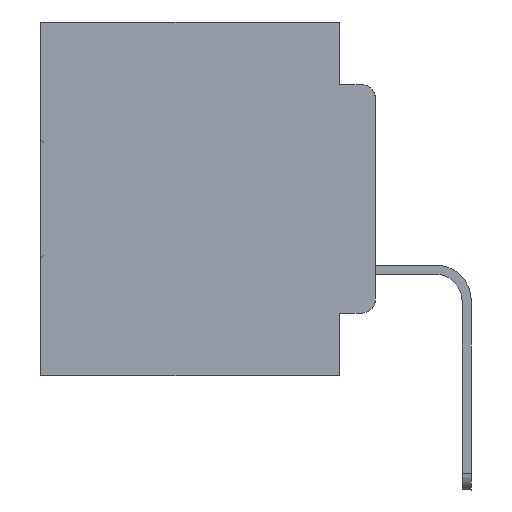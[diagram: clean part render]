
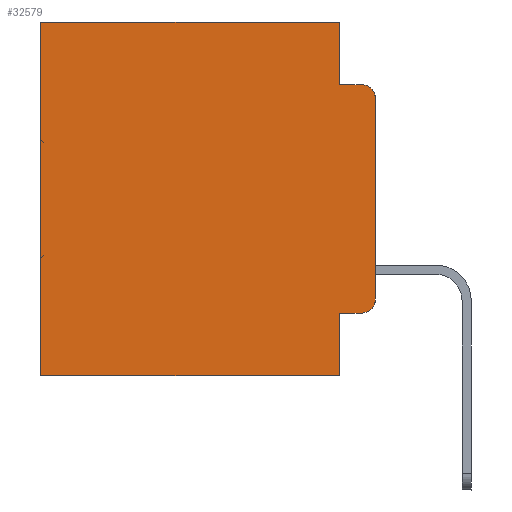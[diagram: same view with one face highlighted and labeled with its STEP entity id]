
A CAD part, left-side view. The second image highlights one B-rep face of the part: STEP entity #32579.
In plain terms, the highlighted planar face has unit normal (-1, 0, 0).
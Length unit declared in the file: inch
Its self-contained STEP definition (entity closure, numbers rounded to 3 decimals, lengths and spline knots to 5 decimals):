
#278 = CARTESIAN_POINT ( 'NONE',  ( 0.298, 0., 0. ) ) ;
#355 = EDGE_CURVE ( 'NONE', #19585, #31760, #22378, .T. ) ;
#626 = ORIENTED_EDGE ( 'NONE', *, *, #24325, .T. ) ;
#877 = EDGE_CURVE ( 'NONE', #32521, #30962, #10411, .T. ) ;
#1264 = VECTOR ( 'NONE', #29494, 39.37008 ) ;
#1660 = DIRECTION ( 'NONE',  ( 0., 0., -1. ) ) ;
#1987 = DIRECTION ( 'NONE',  ( -1., 0., 0. ) ) ;
#2666 = CARTESIAN_POINT ( 'NONE',  ( 0.298, 0., 0. ) ) ;
#3188 = ORIENTED_EDGE ( 'NONE', *, *, #12017, .T. ) ;
#3655 = EDGE_CURVE ( 'NONE', #21389, #31760, #29074, .T. ) ;
#5189 = DIRECTION ( 'NONE',  ( 0., 0., -1. ) ) ;
#5774 = VECTOR ( 'NONE', #8723, 39.37008 ) ;
#5936 = VERTEX_POINT ( 'NONE', #6763 ) ;
#6023 = LINE ( 'NONE', #7294, #16768 ) ;
#6763 = CARTESIAN_POINT ( 'NONE',  ( 0.298, 0.473, -0.5 ) ) ;
#7294 = CARTESIAN_POINT ( 'NONE',  ( 0.298, 0., 0. ) ) ;
#7408 = DIRECTION ( 'NONE',  ( 1., 0., 0. ) ) ;
#7575 = VERTEX_POINT ( 'NONE', #22818 ) ;
#8471 = CARTESIAN_POINT ( 'NONE',  ( 0.298, 0.051, -0.4115 ) ) ;
#8699 = EDGE_CURVE ( 'NONE', #19585, #7575, #6023, .T. ) ;
#8723 = DIRECTION ( 'NONE',  ( 0., 0., -1. ) ) ;
#8889 = CARTESIAN_POINT ( 'NONE',  ( 0.298, 0.02, -0.1085 ) ) ;
#9190 = ORIENTED_EDGE ( 'NONE', *, *, #877, .T. ) ;
#9593 = CARTESIAN_POINT ( 'NONE',  ( 0.298, 0., -0.5 ) ) ;
#9748 = AXIS2_PLACEMENT_3D ( 'NONE', #21970, #1987, #1660 ) ;
#10197 = CARTESIAN_POINT ( 'NONE',  ( 0.298, 0.051, 0. ) ) ;
#10310 = DIRECTION ( 'NONE',  ( 0., 0., -1. ) ) ;
#10411 = LINE ( 'NONE', #278, #21538 ) ;
#11334 = ORIENTED_EDGE ( 'NONE', *, *, #18060, .F. ) ;
#11462 = DIRECTION ( 'NONE',  ( 0., 0., -1. ) ) ;
#11574 = DIRECTION ( 'NONE',  ( 0., -1., 0. ) ) ;
#12017 = EDGE_CURVE ( 'NONE', #30499, #7575, #15718, .T. ) ;
#12837 = EDGE_CURVE ( 'NONE', #30962, #5936, #30762, .T. ) ;
#13956 = ORIENTED_EDGE ( 'NONE', *, *, #20355, .F. ) ;
#14721 = CARTESIAN_POINT ( 'NONE',  ( 0.298, 0.051, -0.5 ) ) ;
#15050 = VERTEX_POINT ( 'NONE', #14721 ) ;
#15686 = DIRECTION ( 'NONE',  ( 0., 1., 0. ) ) ;
#15718 = CIRCLE ( 'NONE', #9748, 0.02 ) ;
#15962 = EDGE_CURVE ( 'NONE', #32521, #21389, #18105, .T. ) ;
#15994 = CARTESIAN_POINT ( 'NONE',  ( 0.298, 0., -0.1085 ) ) ;
#16295 = CARTESIAN_POINT ( 'NONE',  ( 0.298, 0.051, 0. ) ) ;
#16624 = CARTESIAN_POINT ( 'NONE',  ( 0.298, 0.051, 0. ) ) ;
#16768 = VECTOR ( 'NONE', #5189, 39.37008 ) ;
#17450 = CARTESIAN_POINT ( 'NONE',  ( 0.298, 0.473, 0. ) ) ;
#18060 = EDGE_CURVE ( 'NONE', #15050, #5936, #26297, .T. ) ;
#18105 = LINE ( 'NONE', #16295, #5774 ) ;
#18401 = CARTESIAN_POINT ( 'NONE',  ( 0.298, 0.473, 0. ) ) ;
#19118 = LINE ( 'NONE', #16624, #1264 ) ;
#19585 = VERTEX_POINT ( 'NONE', #15994 ) ;
#20034 = DIRECTION ( 'NONE',  ( 0., 1., 0. ) ) ;
#20170 = CARTESIAN_POINT ( 'NONE',  ( 0.298, 0.02, -0.4115 ) ) ;
#20345 = VERTEX_POINT ( 'NONE', #26493 ) ;
#20355 = EDGE_CURVE ( 'NONE', #20345, #15050, #19118, .T. ) ;
#21241 = ORIENTED_EDGE ( 'NONE', *, *, #8699, .F. ) ;
#21389 = VERTEX_POINT ( 'NONE', #28656 ) ;
#21464 = DIRECTION ( 'NONE',  ( -1., 0., 0. ) ) ;
#21538 = VECTOR ( 'NONE', #15686, 39.37008 ) ;
#21680 = FACE_OUTER_BOUND ( 'NONE', #28703, .T. ) ;
#21955 = VECTOR ( 'NONE', #11574, 39.37008 ) ;
#21970 = CARTESIAN_POINT ( 'NONE',  ( 0.298, 0.02, -0.3915 ) ) ;
#22127 = CARTESIAN_POINT ( 'NONE',  ( 0.298, 0.051, -0.0885 ) ) ;
#22378 = CIRCLE ( 'NONE', #24631, 0.02 ) ;
#22818 = CARTESIAN_POINT ( 'NONE',  ( 0.298, 0., -0.3915 ) ) ;
#24325 = EDGE_CURVE ( 'NONE', #20345, #30499, #26422, .T. ) ;
#24631 = AXIS2_PLACEMENT_3D ( 'NONE', #8889, #21464, #11462 ) ;
#26297 = LINE ( 'NONE', #9593, #27098 ) ;
#26422 = LINE ( 'NONE', #8471, #30422 ) ;
#26493 = CARTESIAN_POINT ( 'NONE',  ( 0.298, 0.051, -0.4115 ) ) ;
#27098 = VECTOR ( 'NONE', #20034, 39.37008 ) ;
#27568 = ORIENTED_EDGE ( 'NONE', *, *, #3655, .F. ) ;
#27624 = AXIS2_PLACEMENT_3D ( 'NONE', #2666, #7408, #10310 ) ;
#28656 = CARTESIAN_POINT ( 'NONE',  ( 0.298, 0.051, -0.0885 ) ) ;
#28703 = EDGE_LOOP ( 'NONE', ( #21241, #32092, #27568, #29388, #9190, #32062, #11334, #13956, #626, #3188 ) ) ;
#29074 = LINE ( 'NONE', #22127, #21955 ) ;
#29388 = ORIENTED_EDGE ( 'NONE', *, *, #15962, .F. ) ;
#29494 = DIRECTION ( 'NONE',  ( 0., 0., -1. ) ) ;
#29947 = VECTOR ( 'NONE', #30461, 39.37008 ) ;
#30195 = PLANE ( 'NONE',  #27624 ) ;
#30422 = VECTOR ( 'NONE', #31362, 39.37008 ) ;
#30461 = DIRECTION ( 'NONE',  ( 0., 0., -1. ) ) ;
#30499 = VERTEX_POINT ( 'NONE', #20170 ) ;
#30762 = LINE ( 'NONE', #17450, #29947 ) ;
#30962 = VERTEX_POINT ( 'NONE', #18401 ) ;
#31362 = DIRECTION ( 'NONE',  ( 0., -1., 0. ) ) ;
#31760 = VERTEX_POINT ( 'NONE', #32007 ) ;
#32007 = CARTESIAN_POINT ( 'NONE',  ( 0.298, 0.02, -0.0885 ) ) ;
#32062 = ORIENTED_EDGE ( 'NONE', *, *, #12837, .T. ) ;
#32092 = ORIENTED_EDGE ( 'NONE', *, *, #355, .T. ) ;
#32521 = VERTEX_POINT ( 'NONE', #10197 ) ;
#32579 = ADVANCED_FACE ( 'NONE', ( #21680 ), #30195, .F. ) ;
